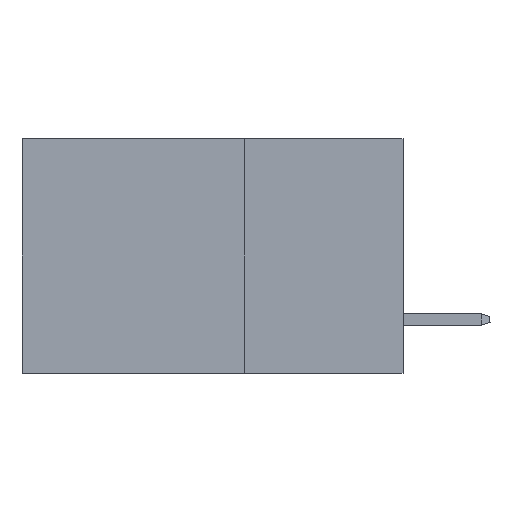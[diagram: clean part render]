
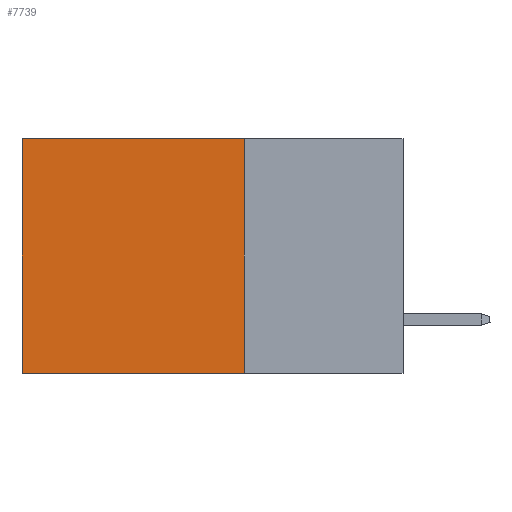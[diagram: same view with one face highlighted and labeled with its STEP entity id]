
A CAD part, left-side view. The second image highlights one B-rep face of the part: STEP entity #7739.
In plain terms, the highlighted planar face has unit normal (-1, 0, 0).
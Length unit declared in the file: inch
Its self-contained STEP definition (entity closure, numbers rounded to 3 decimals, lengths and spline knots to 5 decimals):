
#1665 = ORIENTED_EDGE ( 'NONE', *, *, #19146, .F. ) ;
#2428 = FACE_OUTER_BOUND ( 'NONE', #13962, .T. ) ;
#3444 = CARTESIAN_POINT ( 'NONE',  ( 0.2875, 0.6, 0. ) ) ;
#6868 = EDGE_CURVE ( 'NONE', #30924, #31852, #17582, .T. ) ;
#7739 = ADVANCED_FACE ( 'NONE', ( #2428 ), #35575, .F. ) ;
#11325 = ORIENTED_EDGE ( 'NONE', *, *, #6868, .F. ) ;
#12605 = LINE ( 'NONE', #26956, #16810 ) ;
#13182 = ORIENTED_EDGE ( 'NONE', *, *, #14044, .T. ) ;
#13593 = CARTESIAN_POINT ( 'NONE',  ( 0.2875, 0.25, 0. ) ) ;
#13962 = EDGE_LOOP ( 'NONE', ( #32263, #1665, #11325, #13182 ) ) ;
#14044 = EDGE_CURVE ( 'NONE', #30924, #42805, #35317, .T. ) ;
#16143 = DIRECTION ( 'NONE',  ( 0., 1., 0. ) ) ;
#16810 = VECTOR ( 'NONE', #16143, 39.37008 ) ;
#17582 = LINE ( 'NONE', #28614, #39624 ) ;
#18036 = DIRECTION ( 'NONE',  ( 0., 0., -1. ) ) ;
#19146 = EDGE_CURVE ( 'NONE', #31852, #28063, #12605, .T. ) ;
#20395 = AXIS2_PLACEMENT_3D ( 'NONE', #38392, #42851, #35337 ) ;
#20746 = CARTESIAN_POINT ( 'NONE',  ( 0.2875, 0.25, 0. ) ) ;
#26358 = CARTESIAN_POINT ( 'NONE',  ( 0.2875, 0.6, -0.37 ) ) ;
#26805 = DIRECTION ( 'NONE',  ( 0., 0., -1. ) ) ;
#26956 = CARTESIAN_POINT ( 'NONE',  ( 0.2875, 0.25, -0.37 ) ) ;
#27017 = VECTOR ( 'NONE', #26805, 39.37008 ) ;
#28063 = VERTEX_POINT ( 'NONE', #26358 ) ;
#28614 = CARTESIAN_POINT ( 'NONE',  ( 0.2875, 0.25, 0. ) ) ;
#30027 = VECTOR ( 'NONE', #46131, 39.37008 ) ;
#30924 = VERTEX_POINT ( 'NONE', #13593 ) ;
#31130 = CARTESIAN_POINT ( 'NONE',  ( 0.2875, 0.25, -0.37 ) ) ;
#31852 = VERTEX_POINT ( 'NONE', #31130 ) ;
#32263 = ORIENTED_EDGE ( 'NONE', *, *, #36365, .T. ) ;
#34316 = LINE ( 'NONE', #44899, #27017 ) ;
#35317 = LINE ( 'NONE', #20746, #30027 ) ;
#35337 = DIRECTION ( 'NONE',  ( 0., 0., -1. ) ) ;
#35575 = PLANE ( 'NONE',  #20395 ) ;
#36365 = EDGE_CURVE ( 'NONE', #42805, #28063, #34316, .T. ) ;
#38392 = CARTESIAN_POINT ( 'NONE',  ( 0.2875, 0.25, 0. ) ) ;
#39624 = VECTOR ( 'NONE', #18036, 39.37008 ) ;
#42805 = VERTEX_POINT ( 'NONE', #3444 ) ;
#42851 = DIRECTION ( 'NONE',  ( 1., 0., 0. ) ) ;
#44899 = CARTESIAN_POINT ( 'NONE',  ( 0.2875, 0.6, 0. ) ) ;
#46131 = DIRECTION ( 'NONE',  ( 0., 1., 0. ) ) ;
